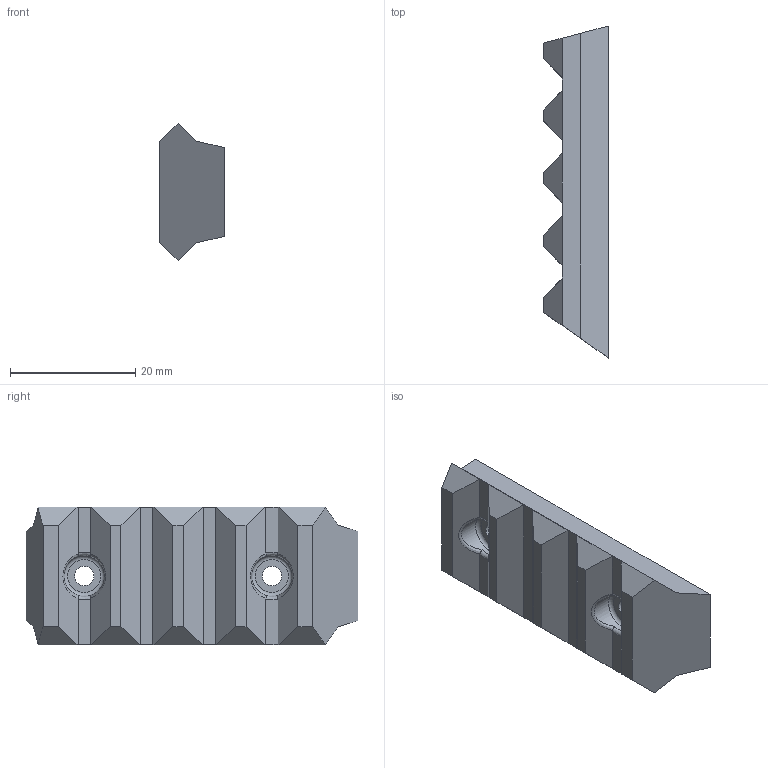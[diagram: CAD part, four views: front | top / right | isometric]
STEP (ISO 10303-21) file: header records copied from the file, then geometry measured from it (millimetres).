
FILE_DESCRIPTION(/* description */ (''),/* implementation_level */ '2;1');
FILE_NAME(/* name */ 'rail xxx fixed.stp',/* time_stamp */ '2021-02-14T02:27:32+02:00',/* author */ (''),/* organization */ (''),/* preprocessor_version */ 'ST-DEVELOPER v15.2',/* originating_system */ 'Autodesk Translator Framework v2.0.0.5431',/* authorisation */ '');
FILE_SCHEMA (('AUTOMOTIVE_DESIGN { 1 0 10303 214 3 1 1 }'));
Length unit declared in the file: centimetre
Products named in the file (1): stock lock
Bounding box: 10.34 x 53.04 x 22.05 mm (x, y, z)
Volume: 7250.4 mm3; surface area: 3383.5 mm2
Topology: 1 solids, 1 shells, 52 faces, 132 edges, 82 vertices
Faces by surface type: plane 38, torus 6, bspline 4, cylinder 4
Full cylindrical faces by diameter (mm): 3.1 x2, 6.5 x2
Entity records: 1740 total; most frequent: CARTESIAN_POINT 538, ORIENTED_EDGE 248, DIRECTION 222, EDGE_CURVE 124, LINE 84, VECTOR 84, VERTEX_POINT 80, AXIS2_PLACEMENT_3D 69
